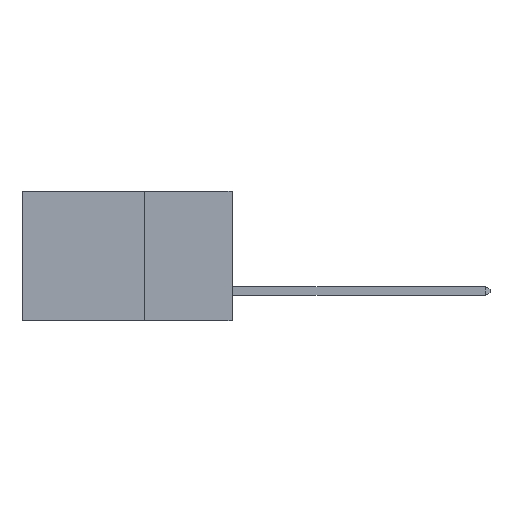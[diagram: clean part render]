
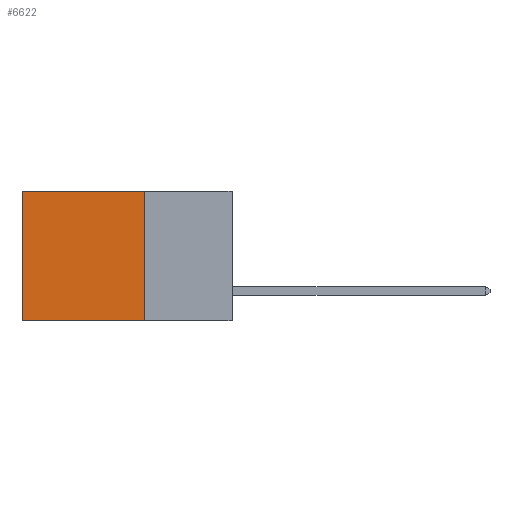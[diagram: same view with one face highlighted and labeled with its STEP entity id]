
A CAD part, left-side view. The second image highlights one B-rep face of the part: STEP entity #6622.
In plain terms, the highlighted planar face has unit normal (-1, 0, 0).
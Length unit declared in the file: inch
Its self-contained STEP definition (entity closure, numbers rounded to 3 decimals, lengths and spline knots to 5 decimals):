
#203 = DIRECTION ( 'NONE',  ( 0., 0., -1. ) ) ;
#503 = EDGE_LOOP ( 'NONE', ( #5074, #11970, #1845, #9453 ) ) ;
#747 = CARTESIAN_POINT ( 'NONE',  ( 0.2875, 0.25, 0. ) ) ;
#1007 = PLANE ( 'NONE',  #6400 ) ;
#1845 = ORIENTED_EDGE ( 'NONE', *, *, #2018, .F. ) ;
#1887 = CARTESIAN_POINT ( 'NONE',  ( 0.2875, 0.25, -0.37 ) ) ;
#2018 = EDGE_CURVE ( 'NONE', #6515, #6619, #13131, .T. ) ;
#2045 = CARTESIAN_POINT ( 'NONE',  ( 0.2875, 0.25, -0.37 ) ) ;
#2937 = CARTESIAN_POINT ( 'NONE',  ( 0.2875, 0.25, 0. ) ) ;
#2992 = VECTOR ( 'NONE', #8135, 39.37008 ) ;
#3023 = EDGE_CURVE ( 'NONE', #11171, #3319, #7730, .T. ) ;
#3319 = VERTEX_POINT ( 'NONE', #8038 ) ;
#3854 = CARTESIAN_POINT ( 'NONE',  ( 0.2875, 0.25, 0. ) ) ;
#4391 = LINE ( 'NONE', #1887, #9945 ) ;
#4416 = CARTESIAN_POINT ( 'NONE',  ( 0.2875, 0.6, 0. ) ) ;
#4430 = CARTESIAN_POINT ( 'NONE',  ( 0.2875, 0.6, 0. ) ) ;
#5074 = ORIENTED_EDGE ( 'NONE', *, *, #3023, .T. ) ;
#5292 = VECTOR ( 'NONE', #10123, 39.37008 ) ;
#5295 = DIRECTION ( 'NONE',  ( 1., 0., 0. ) ) ;
#5872 = EDGE_CURVE ( 'NONE', #6515, #11171, #13345, .T. ) ;
#6400 = AXIS2_PLACEMENT_3D ( 'NONE', #9418, #5295, #12469 ) ;
#6515 = VERTEX_POINT ( 'NONE', #2937 ) ;
#6619 = VERTEX_POINT ( 'NONE', #2045 ) ;
#6622 = ADVANCED_FACE ( 'NONE', ( #13167 ), #1007, .F. ) ;
#7730 = LINE ( 'NONE', #4416, #10122 ) ;
#8038 = CARTESIAN_POINT ( 'NONE',  ( 0.2875, 0.6, -0.37 ) ) ;
#8135 = DIRECTION ( 'NONE',  ( 0., 1., 0. ) ) ;
#9418 = CARTESIAN_POINT ( 'NONE',  ( 0.2875, 0.25, 0. ) ) ;
#9453 = ORIENTED_EDGE ( 'NONE', *, *, #5872, .T. ) ;
#9945 = VECTOR ( 'NONE', #12278, 39.37008 ) ;
#10122 = VECTOR ( 'NONE', #203, 39.37008 ) ;
#10123 = DIRECTION ( 'NONE',  ( 0., 0., -1. ) ) ;
#10877 = EDGE_CURVE ( 'NONE', #6619, #3319, #4391, .T. ) ;
#11171 = VERTEX_POINT ( 'NONE', #4430 ) ;
#11970 = ORIENTED_EDGE ( 'NONE', *, *, #10877, .F. ) ;
#12278 = DIRECTION ( 'NONE',  ( 0., 1., 0. ) ) ;
#12469 = DIRECTION ( 'NONE',  ( 0., 0., -1. ) ) ;
#13131 = LINE ( 'NONE', #3854, #5292 ) ;
#13167 = FACE_OUTER_BOUND ( 'NONE', #503, .T. ) ;
#13345 = LINE ( 'NONE', #747, #2992 ) ;
